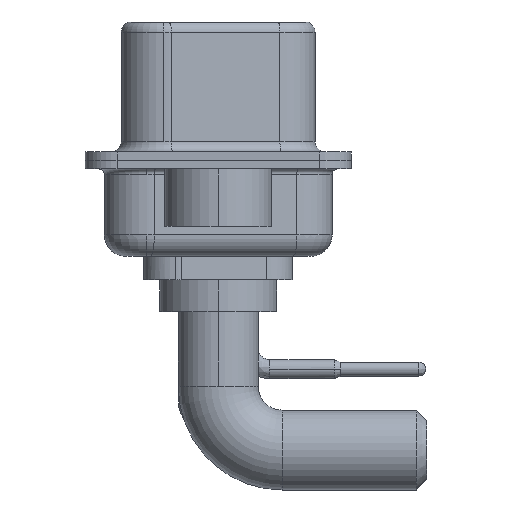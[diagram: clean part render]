
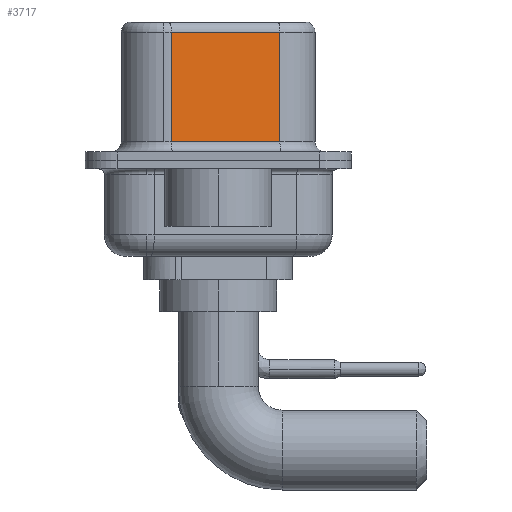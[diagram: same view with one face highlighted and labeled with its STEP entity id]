
A CAD part, left-side view. The second image highlights one B-rep face of the part: STEP entity #3717.
In plain terms, the highlighted planar face has unit normal (-0.985, -0.174, 0).
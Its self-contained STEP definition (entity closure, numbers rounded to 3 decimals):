
#596 = CARTESIAN_POINT ( 'NONE',  ( 3.68, 2.203, 6.52 ) ) ;
#917 = DIRECTION ( 'NONE',  ( 0., 0., -1. ) ) ;
#1814 = CARTESIAN_POINT ( 'NONE',  ( 4.58, -2.897, 6.02 ) ) ;
#2596 = ORIENTED_EDGE ( 'NONE', *, *, #16548, .T. ) ;
#3481 = VECTOR ( 'NONE', #13192, 1000. ) ;
#3717 = ADVANCED_FACE ( 'NONE', ( #20637 ), #15405, .F. ) ;
#4286 = ORIENTED_EDGE ( 'NONE', *, *, #17849, .F. ) ;
#4856 = CARTESIAN_POINT ( 'NONE',  ( 4.58, -2.897, 6.52 ) ) ;
#4905 = CARTESIAN_POINT ( 'NONE',  ( 4.58, -2.897, 6.52 ) ) ;
#5625 = EDGE_CURVE ( 'NONE', #8041, #15147, #10222, .T. ) ;
#5631 = CARTESIAN_POINT ( 'NONE',  ( 4.58, -2.897, 6.02 ) ) ;
#5762 = DIRECTION ( 'NONE',  ( 0.174, -0.985, 0. ) ) ;
#6573 = EDGE_CURVE ( 'NONE', #20159, #8041, #19656, .T. ) ;
#7540 = VECTOR ( 'NONE', #5762, 1000. ) ;
#8034 = CARTESIAN_POINT ( 'NONE',  ( 4.58, -2.897, 0.9 ) ) ;
#8041 = VERTEX_POINT ( 'NONE', #12583 ) ;
#8114 = VECTOR ( 'NONE', #12474, 1000. ) ;
#8360 = DIRECTION ( 'NONE',  ( -0.174, 0.985, 0. ) ) ;
#8823 = LINE ( 'NONE', #1814, #8114 ) ;
#10222 = LINE ( 'NONE', #22400, #7540 ) ;
#11423 = CARTESIAN_POINT ( 'NONE',  ( 3.68, 2.203, 6.02 ) ) ;
#11773 = DIRECTION ( 'NONE',  ( 0.985, 0.174, 0. ) ) ;
#12474 = DIRECTION ( 'NONE',  ( -0.174, 0.985, 0. ) ) ;
#12583 = CARTESIAN_POINT ( 'NONE',  ( 3.68, 2.203, 0.9 ) ) ;
#13192 = DIRECTION ( 'NONE',  ( 0., 0., -1. ) ) ;
#15147 = VERTEX_POINT ( 'NONE', #8034 ) ;
#15405 = PLANE ( 'NONE',  #19421 ) ;
#15600 = VECTOR ( 'NONE', #917, 1000. ) ;
#15778 = VERTEX_POINT ( 'NONE', #5631 ) ;
#16548 = EDGE_CURVE ( 'NONE', #15778, #20159, #8823, .T. ) ;
#17849 = EDGE_CURVE ( 'NONE', #15778, #15147, #20445, .T. ) ;
#18428 = ORIENTED_EDGE ( 'NONE', *, *, #6573, .T. ) ;
#19421 = AXIS2_PLACEMENT_3D ( 'NONE', #4856, #11773, #8360 ) ;
#19656 = LINE ( 'NONE', #596, #15600 ) ;
#20159 = VERTEX_POINT ( 'NONE', #11423 ) ;
#20445 = LINE ( 'NONE', #4905, #3481 ) ;
#20637 = FACE_OUTER_BOUND ( 'NONE', #21214, .T. ) ;
#20914 = ORIENTED_EDGE ( 'NONE', *, *, #5625, .T. ) ;
#21214 = EDGE_LOOP ( 'NONE', ( #4286, #2596, #18428, #20914 ) ) ;
#22400 = CARTESIAN_POINT ( 'NONE',  ( 4.58, -2.897, 0.9 ) ) ;
